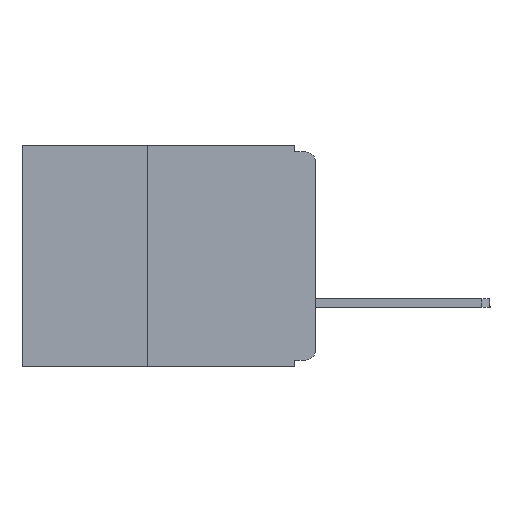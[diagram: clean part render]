
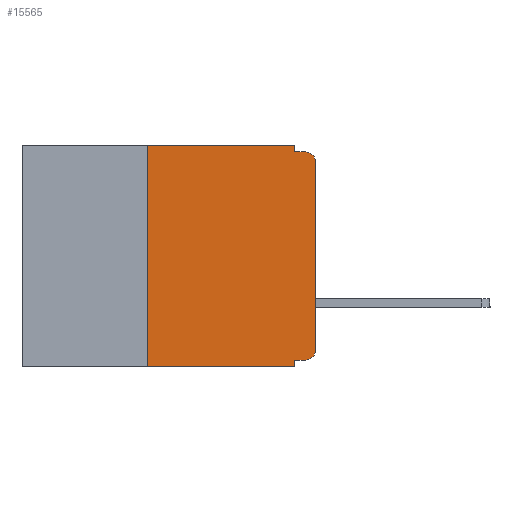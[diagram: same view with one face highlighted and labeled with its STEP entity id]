
A CAD part, left-side view. The second image highlights one B-rep face of the part: STEP entity #15565.
In plain terms, the highlighted planar face has unit normal (-1, 0, 0).
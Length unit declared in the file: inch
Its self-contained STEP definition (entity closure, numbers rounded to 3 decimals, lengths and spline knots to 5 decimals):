
#118 = EDGE_CURVE ( 'NONE', #10169, #22947, #15313, .T. ) ;
#502 = CARTESIAN_POINT ( 'NONE',  ( 0., 0.437, 0. ) ) ;
#548 = CARTESIAN_POINT ( 'NONE',  ( 0., 0.437, 0. ) ) ;
#608 = CARTESIAN_POINT ( 'NONE',  ( 0., 0., 0. ) ) ;
#691 = DIRECTION ( 'NONE',  ( 0., 0., 1. ) ) ;
#830 = EDGE_CURVE ( 'NONE', #7931, #24289, #11867, .T. ) ;
#835 = EDGE_CURVE ( 'NONE', #1863, #10169, #5979, .T. ) ;
#855 = VERTEX_POINT ( 'NONE', #25015 ) ;
#1223 = ORIENTED_EDGE ( 'NONE', *, *, #19363, .T. ) ;
#1863 = VERTEX_POINT ( 'NONE', #13661 ) ;
#1884 = ORIENTED_EDGE ( 'NONE', *, *, #8884, .F. ) ;
#2562 = DIRECTION ( 'NONE',  ( 0., 0., -1. ) ) ;
#2586 = DIRECTION ( 'NONE',  ( 0., 0., -1. ) ) ;
#2603 = DIRECTION ( 'NONE',  ( 0., -1., 0. ) ) ;
#2977 = CARTESIAN_POINT ( 'NONE',  ( 0., 0.031, -0.32 ) ) ;
#3252 = ORIENTED_EDGE ( 'NONE', *, *, #13652, .T. ) ;
#3270 = EDGE_CURVE ( 'NONE', #855, #12408, #14557, .T. ) ;
#3520 = ORIENTED_EDGE ( 'NONE', *, *, #118, .F. ) ;
#3577 = VERTEX_POINT ( 'NONE', #22327 ) ;
#3584 = DIRECTION ( 'NONE',  ( 0., 0., 1. ) ) ;
#3747 = CARTESIAN_POINT ( 'NONE',  ( 0., 0., -0.025 ) ) ;
#3859 = CARTESIAN_POINT ( 'NONE',  ( 0., 0.031, -0.33 ) ) ;
#4136 = CARTESIAN_POINT ( 'NONE',  ( 0., 0., -0.32 ) ) ;
#4155 = VECTOR ( 'NONE', #5227, 39.37008 ) ;
#4455 = CIRCLE ( 'NONE', #23217, 0.015 ) ;
#5227 = DIRECTION ( 'NONE',  ( 0., 0., -1. ) ) ;
#5299 = ORIENTED_EDGE ( 'NONE', *, *, #14868, .T. ) ;
#5411 = LINE ( 'NONE', #22713, #10679 ) ;
#5495 = ORIENTED_EDGE ( 'NONE', *, *, #8536, .T. ) ;
#5570 = CARTESIAN_POINT ( 'NONE',  ( 0., 0., -0.305 ) ) ;
#5979 = LINE ( 'NONE', #4136, #11257 ) ;
#6363 = CARTESIAN_POINT ( 'NONE',  ( 0., 0.015, -0.025 ) ) ;
#6471 = PLANE ( 'NONE',  #16509 ) ;
#6716 = CIRCLE ( 'NONE', #10672, 0.015 ) ;
#7931 = VERTEX_POINT ( 'NONE', #10176 ) ;
#8351 = DIRECTION ( 'NONE',  ( 0., 0., -1. ) ) ;
#8536 = EDGE_CURVE ( 'NONE', #9735, #18444, #9176, .T. ) ;
#8884 = EDGE_CURVE ( 'NONE', #3577, #7931, #21524, .T. ) ;
#9176 = LINE ( 'NONE', #608, #19088 ) ;
#9735 = VERTEX_POINT ( 'NONE', #5570 ) ;
#9851 = CARTESIAN_POINT ( 'NONE',  ( 0., 0.25, 0. ) ) ;
#9982 = VECTOR ( 'NONE', #2603, 39.37008 ) ;
#10169 = VERTEX_POINT ( 'NONE', #2977 ) ;
#10176 = CARTESIAN_POINT ( 'NONE',  ( 0., 0.031, -0.01 ) ) ;
#10215 = CARTESIAN_POINT ( 'NONE',  ( 0., 0.015, -0.305 ) ) ;
#10459 = CARTESIAN_POINT ( 'NONE',  ( 0., 0.031, 0. ) ) ;
#10672 = AXIS2_PLACEMENT_3D ( 'NONE', #6363, #20185, #8351 ) ;
#10679 = VECTOR ( 'NONE', #12899, 39.37008 ) ;
#11257 = VECTOR ( 'NONE', #25068, 39.37008 ) ;
#11867 = LINE ( 'NONE', #22315, #21733 ) ;
#12217 = DIRECTION ( 'NONE',  ( 0., 0., -1. ) ) ;
#12408 = VERTEX_POINT ( 'NONE', #9851 ) ;
#12458 = CARTESIAN_POINT ( 'NONE',  ( 0., 0.031, -0.33 ) ) ;
#12788 = ORIENTED_EDGE ( 'NONE', *, *, #3270, .F. ) ;
#12899 = DIRECTION ( 'NONE',  ( 0., -1., 0. ) ) ;
#13453 = CARTESIAN_POINT ( 'NONE',  ( 0., 0.25, -0.33 ) ) ;
#13590 = DIRECTION ( 'NONE',  ( 0., -1., 0. ) ) ;
#13652 = EDGE_CURVE ( 'NONE', #18444, #24289, #6716, .T. ) ;
#13661 = CARTESIAN_POINT ( 'NONE',  ( 0., 0.015, -0.32 ) ) ;
#14426 = DIRECTION ( 'NONE',  ( 1., 0., 0. ) ) ;
#14557 = LINE ( 'NONE', #13453, #19184 ) ;
#14742 = ORIENTED_EDGE ( 'NONE', *, *, #835, .F. ) ;
#14868 = EDGE_CURVE ( 'NONE', #1863, #9735, #4455, .T. ) ;
#14891 = CARTESIAN_POINT ( 'NONE',  ( 0., 0.015, -0.01 ) ) ;
#15267 = LINE ( 'NONE', #502, #9982 ) ;
#15313 = LINE ( 'NONE', #3859, #4155 ) ;
#15460 = EDGE_LOOP ( 'NONE', ( #5495, #3252, #25285, #1884, #18892, #12788, #1223, #3520, #14742, #5299 ) ) ;
#15565 = ADVANCED_FACE ( 'NONE', ( #23842 ), #6471, .F. ) ;
#16283 = VECTOR ( 'NONE', #2586, 39.37008 ) ;
#16509 = AXIS2_PLACEMENT_3D ( 'NONE', #548, #14426, #2562 ) ;
#18444 = VERTEX_POINT ( 'NONE', #3747 ) ;
#18892 = ORIENTED_EDGE ( 'NONE', *, *, #20198, .F. ) ;
#19088 = VECTOR ( 'NONE', #691, 39.37008 ) ;
#19184 = VECTOR ( 'NONE', #3584, 39.37008 ) ;
#19363 = EDGE_CURVE ( 'NONE', #855, #22947, #5411, .T. ) ;
#20185 = DIRECTION ( 'NONE',  ( -1., 0., 0. ) ) ;
#20198 = EDGE_CURVE ( 'NONE', #12408, #3577, #15267, .T. ) ;
#21524 = LINE ( 'NONE', #10459, #16283 ) ;
#21733 = VECTOR ( 'NONE', #13590, 39.37008 ) ;
#22315 = CARTESIAN_POINT ( 'NONE',  ( 0., 0., -0.01 ) ) ;
#22327 = CARTESIAN_POINT ( 'NONE',  ( 0., 0.031, 0. ) ) ;
#22713 = CARTESIAN_POINT ( 'NONE',  ( 0., 0.437, -0.33 ) ) ;
#22947 = VERTEX_POINT ( 'NONE', #12458 ) ;
#23217 = AXIS2_PLACEMENT_3D ( 'NONE', #10215, #23982, #12217 ) ;
#23842 = FACE_OUTER_BOUND ( 'NONE', #15460, .T. ) ;
#23982 = DIRECTION ( 'NONE',  ( -1., 0., 0. ) ) ;
#24289 = VERTEX_POINT ( 'NONE', #14891 ) ;
#25015 = CARTESIAN_POINT ( 'NONE',  ( 0., 0.25, -0.33 ) ) ;
#25068 = DIRECTION ( 'NONE',  ( 0., 1., 0. ) ) ;
#25285 = ORIENTED_EDGE ( 'NONE', *, *, #830, .F. ) ;
